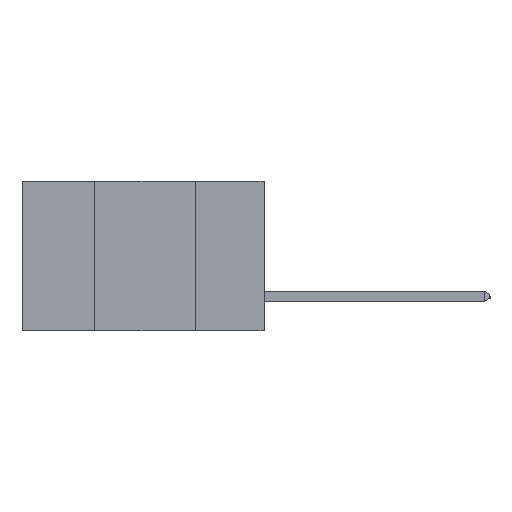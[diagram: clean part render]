
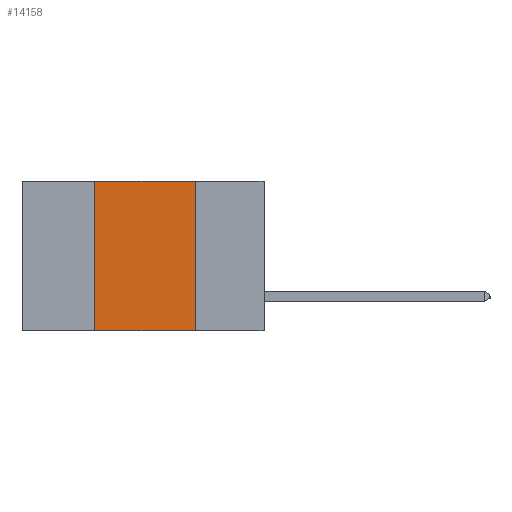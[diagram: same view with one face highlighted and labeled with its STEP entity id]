
A CAD part, left-side view. The second image highlights one B-rep face of the part: STEP entity #14158.
In plain terms, the highlighted planar face has unit normal (-1, 0, 0).
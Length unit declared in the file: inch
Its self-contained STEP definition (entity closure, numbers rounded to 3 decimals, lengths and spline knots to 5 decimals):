
#1126 = ORIENTED_EDGE ( 'NONE', *, *, #17138, .T. ) ;
#2091 = CARTESIAN_POINT ( 'NONE',  ( 0., 0.17, 0. ) ) ;
#2248 = ORIENTED_EDGE ( 'NONE', *, *, #9618, .F. ) ;
#2547 = CARTESIAN_POINT ( 'NONE',  ( 0., 0.17, -0.37 ) ) ;
#4157 = DIRECTION ( 'NONE',  ( 0., 0., 1. ) ) ;
#5401 = EDGE_LOOP ( 'NONE', ( #2248, #8548, #11774, #1126 ) ) ;
#5459 = CARTESIAN_POINT ( 'NONE',  ( 0., 0.6, 0. ) ) ;
#6524 = LINE ( 'NONE', #13607, #13944 ) ;
#7119 = CARTESIAN_POINT ( 'NONE',  ( 0., 0.42, 0. ) ) ;
#7745 = DIRECTION ( 'NONE',  ( 0., -1., 0. ) ) ;
#8548 = ORIENTED_EDGE ( 'NONE', *, *, #16136, .F. ) ;
#9618 = EDGE_CURVE ( 'NONE', #14240, #16258, #11263, .T. ) ;
#9988 = AXIS2_PLACEMENT_3D ( 'NONE', #5459, #18839, #10037 ) ;
#10037 = DIRECTION ( 'NONE',  ( 0., 0., -1. ) ) ;
#10145 = VECTOR ( 'NONE', #4157, 39.37008 ) ;
#10608 = LINE ( 'NONE', #7119, #10145 ) ;
#11263 = LINE ( 'NONE', #2091, #14654 ) ;
#11509 = VECTOR ( 'NONE', #15865, 39.37008 ) ;
#11536 = CARTESIAN_POINT ( 'NONE',  ( 0., 0.6, 0. ) ) ;
#11544 = VERTEX_POINT ( 'NONE', #11749 ) ;
#11749 = CARTESIAN_POINT ( 'NONE',  ( 0., 0.42, -0.37 ) ) ;
#11774 = ORIENTED_EDGE ( 'NONE', *, *, #18484, .F. ) ;
#13071 = CARTESIAN_POINT ( 'NONE',  ( 0., 0.17, 0. ) ) ;
#13607 = CARTESIAN_POINT ( 'NONE',  ( 0., 0.6, -0.37 ) ) ;
#13944 = VECTOR ( 'NONE', #7745, 39.37008 ) ;
#14158 = ADVANCED_FACE ( 'NONE', ( #16868 ), #14370, .F. ) ;
#14240 = VERTEX_POINT ( 'NONE', #13071 ) ;
#14370 = PLANE ( 'NONE',  #9988 ) ;
#14432 = CARTESIAN_POINT ( 'NONE',  ( 0., 0.42, 0. ) ) ;
#14654 = VECTOR ( 'NONE', #18697, 39.37008 ) ;
#15835 = LINE ( 'NONE', #11536, #11509 ) ;
#15865 = DIRECTION ( 'NONE',  ( 0., -1., 0. ) ) ;
#16136 = EDGE_CURVE ( 'NONE', #18408, #14240, #15835, .T. ) ;
#16258 = VERTEX_POINT ( 'NONE', #2547 ) ;
#16868 = FACE_OUTER_BOUND ( 'NONE', #5401, .T. ) ;
#17138 = EDGE_CURVE ( 'NONE', #11544, #16258, #6524, .T. ) ;
#18408 = VERTEX_POINT ( 'NONE', #14432 ) ;
#18484 = EDGE_CURVE ( 'NONE', #11544, #18408, #10608, .T. ) ;
#18697 = DIRECTION ( 'NONE',  ( 0., 0., -1. ) ) ;
#18839 = DIRECTION ( 'NONE',  ( 1., 0., 0. ) ) ;
